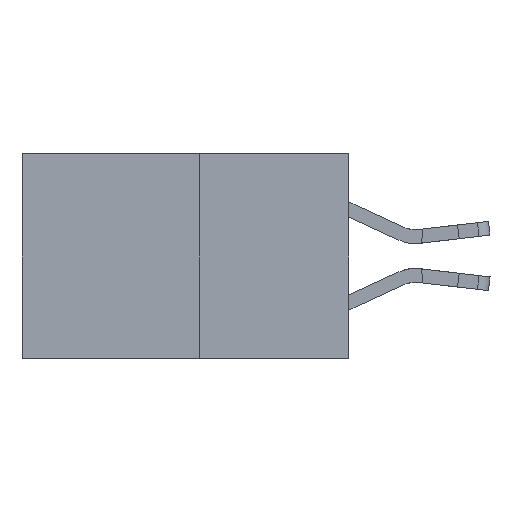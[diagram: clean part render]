
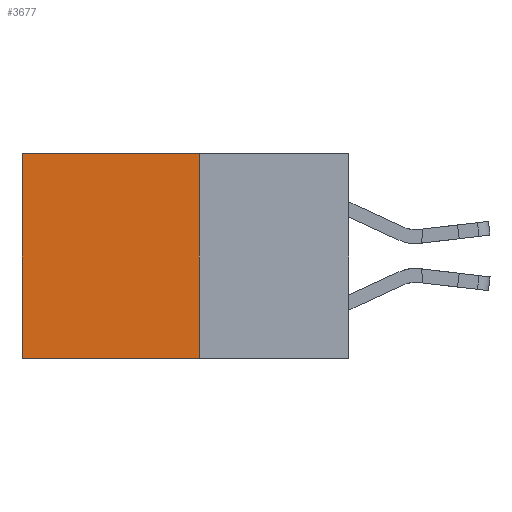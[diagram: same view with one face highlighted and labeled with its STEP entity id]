
A CAD part, left-side view. The second image highlights one B-rep face of the part: STEP entity #3677.
In plain terms, the highlighted planar face has unit normal (-1, 0, 0).
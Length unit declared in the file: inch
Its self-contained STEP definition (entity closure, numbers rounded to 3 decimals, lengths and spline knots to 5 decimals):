
#111 = CARTESIAN_POINT ( 'NONE',  ( 0.277, 0.27, -0.37 ) ) ;
#157 = DIRECTION ( 'NONE',  ( 0., 0., -1. ) ) ;
#3089 = CARTESIAN_POINT ( 'NONE',  ( 0.277, 0.27, -0.37 ) ) ;
#3465 = ORIENTED_EDGE ( 'NONE', *, *, #7216, .F. ) ;
#3677 = ADVANCED_FACE ( 'NONE', ( #14646 ), #9406, .F. ) ;
#3941 = CARTESIAN_POINT ( 'NONE',  ( 0.277, 0.27, 0. ) ) ;
#4105 = ORIENTED_EDGE ( 'NONE', *, *, #17426, .T. ) ;
#5493 = ORIENTED_EDGE ( 'NONE', *, *, #9982, .T. ) ;
#7216 = EDGE_CURVE ( 'NONE', #9182, #10400, #16445, .T. ) ;
#7526 = EDGE_CURVE ( 'NONE', #10400, #10939, #10412, .T. ) ;
#7674 = ORIENTED_EDGE ( 'NONE', *, *, #7526, .F. ) ;
#8855 = EDGE_LOOP ( 'NONE', ( #4105, #7674, #3465, #5493 ) ) ;
#9182 = VERTEX_POINT ( 'NONE', #12155 ) ;
#9306 = DIRECTION ( 'NONE',  ( 0., 0., -1. ) ) ;
#9327 = DIRECTION ( 'NONE',  ( 1., 0., 0. ) ) ;
#9381 = CARTESIAN_POINT ( 'NONE',  ( 0.277, 0.27, -0.37 ) ) ;
#9406 = PLANE ( 'NONE',  #21002 ) ;
#9814 = DIRECTION ( 'NONE',  ( 0., 1., 0. ) ) ;
#9982 = EDGE_CURVE ( 'NONE', #9182, #12807, #15543, .T. ) ;
#10230 = DIRECTION ( 'NONE',  ( 0., 0., -1. ) ) ;
#10400 = VERTEX_POINT ( 'NONE', #3089 ) ;
#10412 = LINE ( 'NONE', #15060, #14539 ) ;
#10872 = VECTOR ( 'NONE', #12728, 39.37008 ) ;
#10939 = VERTEX_POINT ( 'NONE', #13770 ) ;
#11798 = VECTOR ( 'NONE', #157, 39.37008 ) ;
#12155 = CARTESIAN_POINT ( 'NONE',  ( 0.277, 0.27, 0. ) ) ;
#12728 = DIRECTION ( 'NONE',  ( 0., 1., 0. ) ) ;
#12807 = VERTEX_POINT ( 'NONE', #16724 ) ;
#13519 = VECTOR ( 'NONE', #10230, 39.37008 ) ;
#13770 = CARTESIAN_POINT ( 'NONE',  ( 0.277, 0.59, -0.37 ) ) ;
#14539 = VECTOR ( 'NONE', #9814, 39.37008 ) ;
#14646 = FACE_OUTER_BOUND ( 'NONE', #8855, .T. ) ;
#15060 = CARTESIAN_POINT ( 'NONE',  ( 0.277, 0.27, -0.37 ) ) ;
#15543 = LINE ( 'NONE', #3941, #10872 ) ;
#16445 = LINE ( 'NONE', #111, #11798 ) ;
#16724 = CARTESIAN_POINT ( 'NONE',  ( 0.277, 0.59, 0. ) ) ;
#17426 = EDGE_CURVE ( 'NONE', #12807, #10939, #18705, .T. ) ;
#18705 = LINE ( 'NONE', #18971, #13519 ) ;
#18971 = CARTESIAN_POINT ( 'NONE',  ( 0.277, 0.59, -0.37 ) ) ;
#21002 = AXIS2_PLACEMENT_3D ( 'NONE', #9381, #9327, #9306 ) ;
